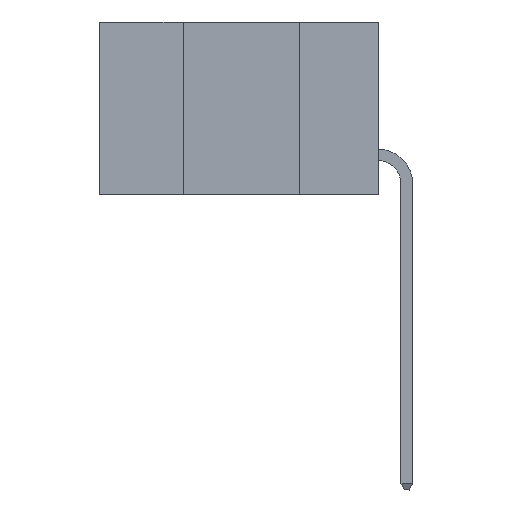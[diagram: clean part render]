
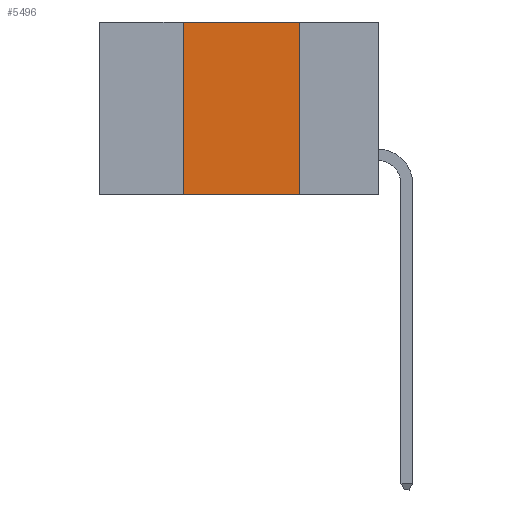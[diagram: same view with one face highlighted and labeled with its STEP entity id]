
A CAD part, left-side view. The second image highlights one B-rep face of the part: STEP entity #5496.
In plain terms, the highlighted planar face has unit normal (-1, 0, 0).
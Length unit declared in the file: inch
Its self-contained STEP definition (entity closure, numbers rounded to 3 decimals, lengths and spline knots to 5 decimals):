
#4 = VECTOR ( 'NONE', #14228, 39.37008 ) ;
#67 = EDGE_CURVE ( 'NONE', #5671, #9670, #2048, .T. ) ;
#1061 = VECTOR ( 'NONE', #5048, 39.37008 ) ;
#1090 = LINE ( 'NONE', #10889, #4 ) ;
#1535 = DIRECTION ( 'NONE',  ( 1., 0., 0. ) ) ;
#1706 = VECTOR ( 'NONE', #7407, 39.37008 ) ;
#2048 = LINE ( 'NONE', #14242, #2679 ) ;
#2125 = DIRECTION ( 'NONE',  ( 0., 0., 1. ) ) ;
#2617 = FACE_OUTER_BOUND ( 'NONE', #7841, .T. ) ;
#2679 = VECTOR ( 'NONE', #2125, 39.37008 ) ;
#3197 = EDGE_CURVE ( 'NONE', #7007, #9431, #1090, .T. ) ;
#3231 = CARTESIAN_POINT ( 'NONE',  ( 0., 0.6, 0. ) ) ;
#5048 = DIRECTION ( 'NONE',  ( 0., -1., 0. ) ) ;
#5496 = ADVANCED_FACE ( 'NONE', ( #2617 ), #7050, .F. ) ;
#5671 = VERTEX_POINT ( 'NONE', #6678 ) ;
#6667 = CARTESIAN_POINT ( 'NONE',  ( 0., 0.17, -0.37 ) ) ;
#6678 = CARTESIAN_POINT ( 'NONE',  ( 0., 0.42, -0.37 ) ) ;
#7007 = VERTEX_POINT ( 'NONE', #9952 ) ;
#7050 = PLANE ( 'NONE',  #12091 ) ;
#7407 = DIRECTION ( 'NONE',  ( 0., -1., 0. ) ) ;
#7745 = EDGE_CURVE ( 'NONE', #9670, #7007, #8739, .T. ) ;
#7841 = EDGE_LOOP ( 'NONE', ( #11407, #13719, #14142, #13987 ) ) ;
#8567 = DIRECTION ( 'NONE',  ( 0., 0., -1. ) ) ;
#8739 = LINE ( 'NONE', #3231, #1061 ) ;
#8875 = EDGE_CURVE ( 'NONE', #5671, #9431, #11829, .T. ) ;
#9431 = VERTEX_POINT ( 'NONE', #6667 ) ;
#9670 = VERTEX_POINT ( 'NONE', #11303 ) ;
#9952 = CARTESIAN_POINT ( 'NONE',  ( 0., 0.17, 0. ) ) ;
#10889 = CARTESIAN_POINT ( 'NONE',  ( 0., 0.17, -0.37 ) ) ;
#11303 = CARTESIAN_POINT ( 'NONE',  ( 0., 0.42, 0. ) ) ;
#11407 = ORIENTED_EDGE ( 'NONE', *, *, #3197, .F. ) ;
#11469 = CARTESIAN_POINT ( 'NONE',  ( 0., 0.6, 0. ) ) ;
#11751 = CARTESIAN_POINT ( 'NONE',  ( 0., 0.6, -0.37 ) ) ;
#11829 = LINE ( 'NONE', #11751, #1706 ) ;
#12091 = AXIS2_PLACEMENT_3D ( 'NONE', #11469, #1535, #8567 ) ;
#13719 = ORIENTED_EDGE ( 'NONE', *, *, #7745, .F. ) ;
#13987 = ORIENTED_EDGE ( 'NONE', *, *, #8875, .T. ) ;
#14142 = ORIENTED_EDGE ( 'NONE', *, *, #67, .F. ) ;
#14228 = DIRECTION ( 'NONE',  ( 0., 0., -1. ) ) ;
#14242 = CARTESIAN_POINT ( 'NONE',  ( 0., 0.42, -0.37 ) ) ;
